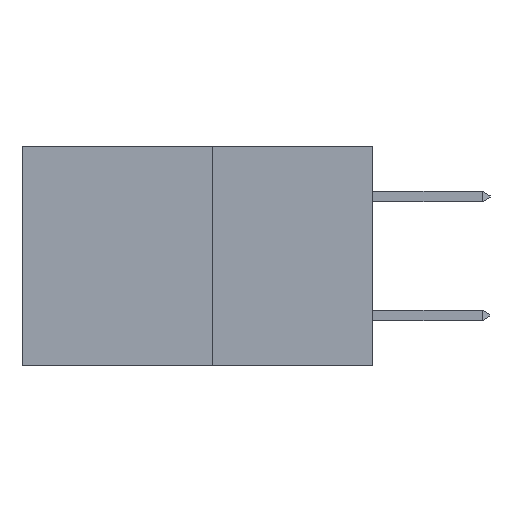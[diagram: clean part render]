
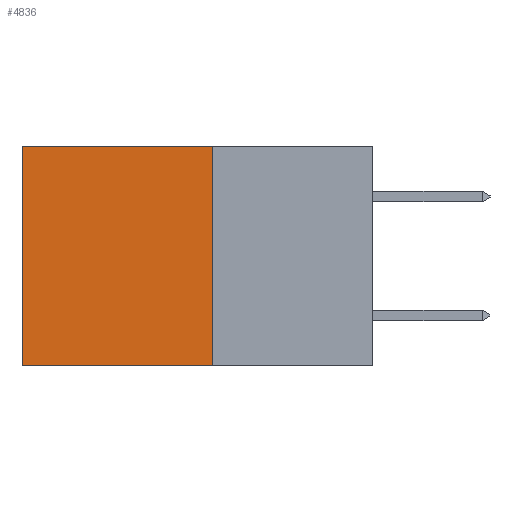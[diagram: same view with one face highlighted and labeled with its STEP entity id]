
A CAD part, left-side view. The second image highlights one B-rep face of the part: STEP entity #4836.
In plain terms, the highlighted planar face has unit normal (-1, 0, 0).
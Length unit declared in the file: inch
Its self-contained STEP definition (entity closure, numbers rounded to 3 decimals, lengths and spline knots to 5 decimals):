
#300 = VERTEX_POINT ( 'NONE', #6967 ) ;
#802 = AXIS2_PLACEMENT_3D ( 'NONE', #6984, #6791, #6873 ) ;
#850 = DIRECTION ( 'NONE',  ( 0., 1., 0. ) ) ;
#975 = ORIENTED_EDGE ( 'NONE', *, *, #3511, .T. ) ;
#1051 = CARTESIAN_POINT ( 'NONE',  ( 0.277, 0.59, 0. ) ) ;
#1323 = CARTESIAN_POINT ( 'NONE',  ( 0.277, 0.27, -0.37 ) ) ;
#1683 = CARTESIAN_POINT ( 'NONE',  ( 0.277, 0.27, -0.37 ) ) ;
#1744 = EDGE_CURVE ( 'NONE', #5058, #4113, #3261, .T. ) ;
#2155 = ORIENTED_EDGE ( 'NONE', *, *, #1744, .F. ) ;
#2411 = EDGE_CURVE ( 'NONE', #300, #5058, #5785, .T. ) ;
#2482 = ORIENTED_EDGE ( 'NONE', *, *, #3845, .T. ) ;
#2519 = FACE_OUTER_BOUND ( 'NONE', #2579, .T. ) ;
#2579 = EDGE_LOOP ( 'NONE', ( #2482, #2155, #8247, #975 ) ) ;
#3261 = LINE ( 'NONE', #1683, #5096 ) ;
#3384 = DIRECTION ( 'NONE',  ( 0., 0., -1. ) ) ;
#3511 = EDGE_CURVE ( 'NONE', #300, #9365, #5133, .T. ) ;
#3845 = EDGE_CURVE ( 'NONE', #9365, #4113, #9988, .T. ) ;
#4113 = VERTEX_POINT ( 'NONE', #4289 ) ;
#4289 = CARTESIAN_POINT ( 'NONE',  ( 0.277, 0.59, -0.37 ) ) ;
#4836 = ADVANCED_FACE ( 'NONE', ( #2519 ), #6342, .F. ) ;
#4901 = VECTOR ( 'NONE', #7123, 39.37008 ) ;
#5058 = VERTEX_POINT ( 'NONE', #7892 ) ;
#5096 = VECTOR ( 'NONE', #850, 39.37008 ) ;
#5133 = LINE ( 'NONE', #5981, #4901 ) ;
#5367 = DIRECTION ( 'NONE',  ( 0., 0., -1. ) ) ;
#5785 = LINE ( 'NONE', #1323, #7579 ) ;
#5981 = CARTESIAN_POINT ( 'NONE',  ( 0.277, 0.27, 0. ) ) ;
#6342 = PLANE ( 'NONE',  #802 ) ;
#6791 = DIRECTION ( 'NONE',  ( 1., 0., 0. ) ) ;
#6873 = DIRECTION ( 'NONE',  ( 0., 0., -1. ) ) ;
#6967 = CARTESIAN_POINT ( 'NONE',  ( 0.277, 0.27, 0. ) ) ;
#6984 = CARTESIAN_POINT ( 'NONE',  ( 0.277, 0.27, -0.37 ) ) ;
#7123 = DIRECTION ( 'NONE',  ( 0., 1., 0. ) ) ;
#7579 = VECTOR ( 'NONE', #3384, 39.37008 ) ;
#7892 = CARTESIAN_POINT ( 'NONE',  ( 0.277, 0.27, -0.37 ) ) ;
#8222 = CARTESIAN_POINT ( 'NONE',  ( 0.277, 0.59, -0.37 ) ) ;
#8247 = ORIENTED_EDGE ( 'NONE', *, *, #2411, .F. ) ;
#9365 = VERTEX_POINT ( 'NONE', #1051 ) ;
#9758 = VECTOR ( 'NONE', #5367, 39.37008 ) ;
#9988 = LINE ( 'NONE', #8222, #9758 ) ;
